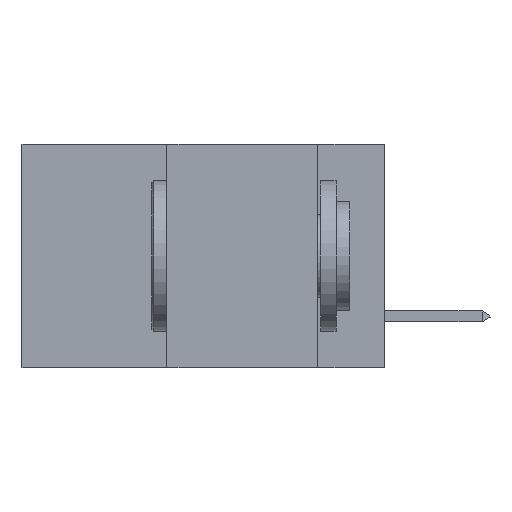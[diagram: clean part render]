
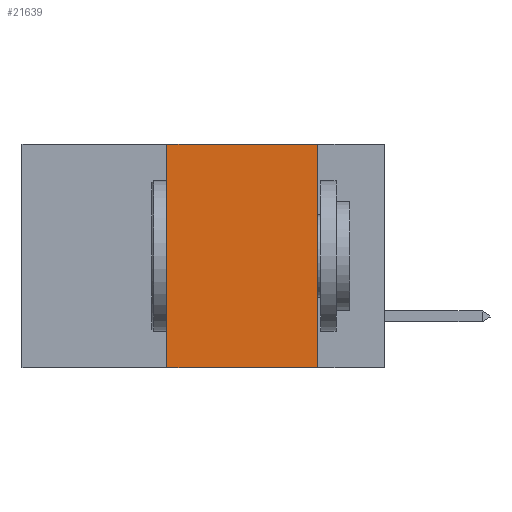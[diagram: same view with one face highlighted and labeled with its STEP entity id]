
A CAD part, left-side view. The second image highlights one B-rep face of the part: STEP entity #21639.
In plain terms, the highlighted planar face has unit normal (-1, 0, 0).
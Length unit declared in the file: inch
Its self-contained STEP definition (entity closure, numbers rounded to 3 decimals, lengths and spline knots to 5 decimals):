
#1041 = CARTESIAN_POINT ( 'NONE',  ( 0., 0.36, 0. ) ) ;
#4314 = EDGE_CURVE ( 'NONE', #26248, #29640, #46063, .T. ) ;
#4431 = ORIENTED_EDGE ( 'NONE', *, *, #27259, .F. ) ;
#5165 = DIRECTION ( 'NONE',  ( 0., -1., 0. ) ) ;
#5246 = CARTESIAN_POINT ( 'NONE',  ( 0., 0.36, -0.37 ) ) ;
#7338 = CARTESIAN_POINT ( 'NONE',  ( 0., 0.6, 0. ) ) ;
#8305 = DIRECTION ( 'NONE',  ( 1., 0., 0. ) ) ;
#9932 = LINE ( 'NONE', #12844, #50707 ) ;
#10605 = CARTESIAN_POINT ( 'NONE',  ( 0., 0.6, 0. ) ) ;
#12837 = CARTESIAN_POINT ( 'NONE',  ( 0., 0.6, -0.37 ) ) ;
#12844 = CARTESIAN_POINT ( 'NONE',  ( 0., 0.11, 0. ) ) ;
#14179 = CARTESIAN_POINT ( 'NONE',  ( 0., 0.36, 0. ) ) ;
#16084 = LINE ( 'NONE', #12837, #33403 ) ;
#16992 = DIRECTION ( 'NONE',  ( 0., 0., -1. ) ) ;
#16998 = VECTOR ( 'NONE', #17796, 39.37008 ) ;
#17796 = DIRECTION ( 'NONE',  ( 0., 0., 1. ) ) ;
#21639 = ADVANCED_FACE ( 'NONE', ( #40187 ), #49721, .F. ) ;
#22407 = VERTEX_POINT ( 'NONE', #41207 ) ;
#23385 = EDGE_LOOP ( 'NONE', ( #4431, #38372, #49850, #48399 ) ) ;
#24532 = EDGE_CURVE ( 'NONE', #29640, #48313, #46556, .T. ) ;
#26248 = VERTEX_POINT ( 'NONE', #5246 ) ;
#26566 = DIRECTION ( 'NONE',  ( 0., -1., 0. ) ) ;
#27053 = DIRECTION ( 'NONE',  ( 0., 0., -1. ) ) ;
#27259 = EDGE_CURVE ( 'NONE', #48313, #22407, #9932, .T. ) ;
#29188 = EDGE_CURVE ( 'NONE', #26248, #22407, #16084, .T. ) ;
#29640 = VERTEX_POINT ( 'NONE', #1041 ) ;
#33403 = VECTOR ( 'NONE', #5165, 39.37008 ) ;
#34169 = CARTESIAN_POINT ( 'NONE',  ( 0., 0.11, 0. ) ) ;
#35050 = AXIS2_PLACEMENT_3D ( 'NONE', #10605, #8305, #27053 ) ;
#36042 = VECTOR ( 'NONE', #26566, 39.37008 ) ;
#38372 = ORIENTED_EDGE ( 'NONE', *, *, #24532, .F. ) ;
#40187 = FACE_OUTER_BOUND ( 'NONE', #23385, .T. ) ;
#41207 = CARTESIAN_POINT ( 'NONE',  ( 0., 0.11, -0.37 ) ) ;
#46063 = LINE ( 'NONE', #14179, #16998 ) ;
#46556 = LINE ( 'NONE', #7338, #36042 ) ;
#48313 = VERTEX_POINT ( 'NONE', #34169 ) ;
#48399 = ORIENTED_EDGE ( 'NONE', *, *, #29188, .T. ) ;
#49721 = PLANE ( 'NONE',  #35050 ) ;
#49850 = ORIENTED_EDGE ( 'NONE', *, *, #4314, .F. ) ;
#50707 = VECTOR ( 'NONE', #16992, 39.37008 ) ;
